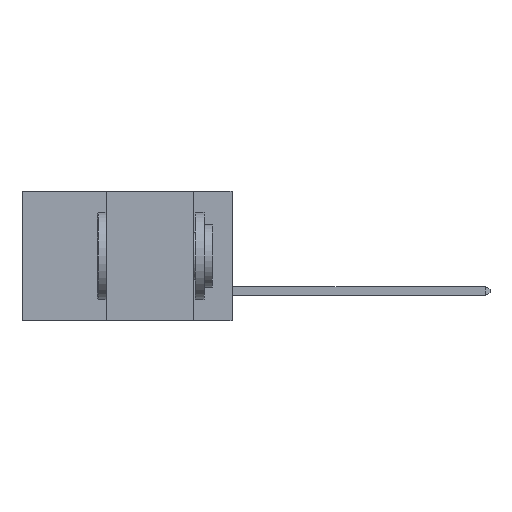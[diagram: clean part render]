
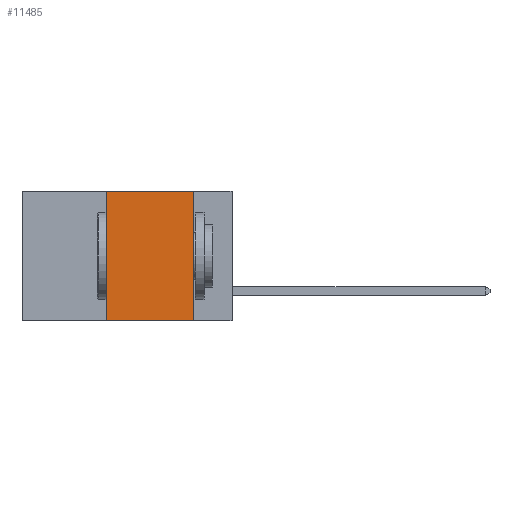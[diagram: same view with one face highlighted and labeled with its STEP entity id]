
A CAD part, left-side view. The second image highlights one B-rep face of the part: STEP entity #11485.
In plain terms, the highlighted planar face has unit normal (-1, 0, 0).
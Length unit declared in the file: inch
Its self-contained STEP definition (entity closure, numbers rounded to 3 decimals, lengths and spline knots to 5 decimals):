
#282 = DIRECTION ( 'NONE',  ( 0., -1., 0. ) ) ;
#627 = DIRECTION ( 'NONE',  ( 0., 0., -1. ) ) ;
#721 = EDGE_CURVE ( 'NONE', #17993, #14398, #11046, .T. ) ;
#1162 = CARTESIAN_POINT ( 'NONE',  ( 0., 0.11, 0. ) ) ;
#1482 = EDGE_CURVE ( 'NONE', #18075, #17993, #13998, .T. ) ;
#2864 = AXIS2_PLACEMENT_3D ( 'NONE', #6478, #20037, #8415 ) ;
#3855 = CARTESIAN_POINT ( 'NONE',  ( 0., 0.11, -0.37 ) ) ;
#4259 = LINE ( 'NONE', #10129, #18477 ) ;
#5394 = EDGE_LOOP ( 'NONE', ( #13587, #24623, #14794, #20023 ) ) ;
#5725 = VECTOR ( 'NONE', #627, 39.37008 ) ;
#5925 = VECTOR ( 'NONE', #13266, 39.37008 ) ;
#6478 = CARTESIAN_POINT ( 'NONE',  ( 0., 0.6, 0. ) ) ;
#8415 = DIRECTION ( 'NONE',  ( 0., 0., -1. ) ) ;
#8513 = CARTESIAN_POINT ( 'NONE',  ( 0., 0.11, 0. ) ) ;
#8905 = VECTOR ( 'NONE', #16104, 39.37008 ) ;
#10129 = CARTESIAN_POINT ( 'NONE',  ( 0., 0.6, -0.37 ) ) ;
#10829 = LINE ( 'NONE', #8513, #5725 ) ;
#11046 = LINE ( 'NONE', #13472, #5925 ) ;
#11168 = EDGE_CURVE ( 'NONE', #18075, #13175, #4259, .T. ) ;
#11485 = ADVANCED_FACE ( 'NONE', ( #20925 ), #14116, .F. ) ;
#12791 = EDGE_CURVE ( 'NONE', #14398, #13175, #10829, .T. ) ;
#13175 = VERTEX_POINT ( 'NONE', #3855 ) ;
#13266 = DIRECTION ( 'NONE',  ( 0., -1., 0. ) ) ;
#13472 = CARTESIAN_POINT ( 'NONE',  ( 0., 0.6, 0. ) ) ;
#13587 = ORIENTED_EDGE ( 'NONE', *, *, #12791, .F. ) ;
#13998 = LINE ( 'NONE', #16279, #8905 ) ;
#14116 = PLANE ( 'NONE',  #2864 ) ;
#14398 = VERTEX_POINT ( 'NONE', #1162 ) ;
#14794 = ORIENTED_EDGE ( 'NONE', *, *, #1482, .F. ) ;
#16104 = DIRECTION ( 'NONE',  ( 0., 0., 1. ) ) ;
#16279 = CARTESIAN_POINT ( 'NONE',  ( 0., 0.36, 0. ) ) ;
#17742 = CARTESIAN_POINT ( 'NONE',  ( 0., 0.36, 0. ) ) ;
#17993 = VERTEX_POINT ( 'NONE', #17742 ) ;
#18075 = VERTEX_POINT ( 'NONE', #19990 ) ;
#18477 = VECTOR ( 'NONE', #282, 39.37008 ) ;
#19990 = CARTESIAN_POINT ( 'NONE',  ( 0., 0.36, -0.37 ) ) ;
#20023 = ORIENTED_EDGE ( 'NONE', *, *, #11168, .T. ) ;
#20037 = DIRECTION ( 'NONE',  ( 1., 0., 0. ) ) ;
#20925 = FACE_OUTER_BOUND ( 'NONE', #5394, .T. ) ;
#24623 = ORIENTED_EDGE ( 'NONE', *, *, #721, .F. ) ;
